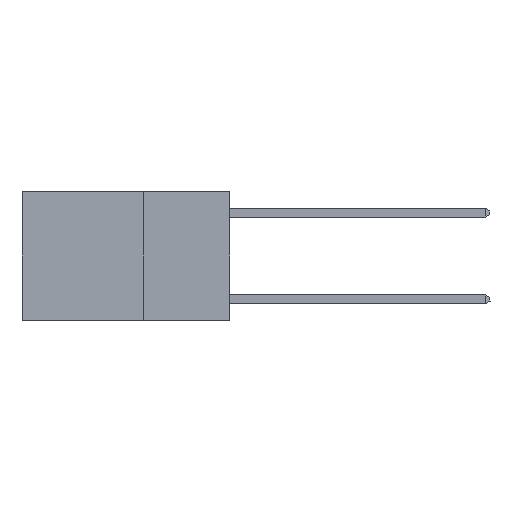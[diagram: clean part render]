
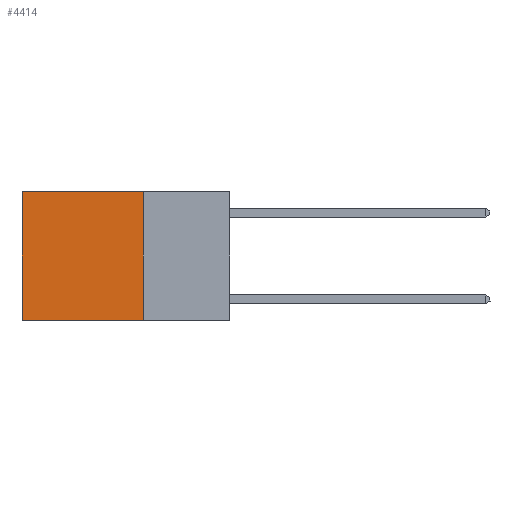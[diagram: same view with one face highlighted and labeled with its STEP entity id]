
A CAD part, left-side view. The second image highlights one B-rep face of the part: STEP entity #4414.
In plain terms, the highlighted planar face has unit normal (-1, 0, 0).
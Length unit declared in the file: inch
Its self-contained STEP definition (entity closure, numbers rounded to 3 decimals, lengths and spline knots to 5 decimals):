
#2287 = EDGE_CURVE ( 'NONE', #24122, #11270, #14135, .T. ) ;
#2678 = EDGE_CURVE ( 'NONE', #27403, #24122, #9421, .T. ) ;
#4101 = AXIS2_PLACEMENT_3D ( 'NONE', #6440, #26783, #15635 ) ;
#4414 = ADVANCED_FACE ( 'NONE', ( #10838 ), #17361, .F. ) ;
#4467 = VECTOR ( 'NONE', #24003, 39.37008 ) ;
#6440 = CARTESIAN_POINT ( 'NONE',  ( 0.2625, 0.25, 0. ) ) ;
#7642 = CARTESIAN_POINT ( 'NONE',  ( 0.2625, 0.25, 0. ) ) ;
#7961 = CARTESIAN_POINT ( 'NONE',  ( 0.2625, 0.6, 0. ) ) ;
#8773 = CARTESIAN_POINT ( 'NONE',  ( 0.2625, 0.25, -0.37 ) ) ;
#9421 = LINE ( 'NONE', #28449, #4467 ) ;
#10534 = EDGE_CURVE ( 'NONE', #18274, #11270, #14956, .T. ) ;
#10838 = FACE_OUTER_BOUND ( 'NONE', #27729, .T. ) ;
#11270 = VERTEX_POINT ( 'NONE', #27602 ) ;
#12934 = LINE ( 'NONE', #20605, #22200 ) ;
#14135 = LINE ( 'NONE', #8773, #26970 ) ;
#14956 = LINE ( 'NONE', #7961, #27405 ) ;
#15513 = ORIENTED_EDGE ( 'NONE', *, *, #2678, .F. ) ;
#15635 = DIRECTION ( 'NONE',  ( 0., 0., -1. ) ) ;
#16086 = DIRECTION ( 'NONE',  ( 0., 1., 0. ) ) ;
#17361 = PLANE ( 'NONE',  #4101 ) ;
#18274 = VERTEX_POINT ( 'NONE', #22081 ) ;
#20605 = CARTESIAN_POINT ( 'NONE',  ( 0.2625, 0.25, 0. ) ) ;
#20937 = ORIENTED_EDGE ( 'NONE', *, *, #10534, .T. ) ;
#22081 = CARTESIAN_POINT ( 'NONE',  ( 0.2625, 0.6, 0. ) ) ;
#22200 = VECTOR ( 'NONE', #16086, 39.37008 ) ;
#23156 = EDGE_CURVE ( 'NONE', #27403, #18274, #12934, .T. ) ;
#24003 = DIRECTION ( 'NONE',  ( 0., 0., -1. ) ) ;
#24122 = VERTEX_POINT ( 'NONE', #26288 ) ;
#24242 = DIRECTION ( 'NONE',  ( 0., 0., -1. ) ) ;
#26138 = ORIENTED_EDGE ( 'NONE', *, *, #2287, .F. ) ;
#26288 = CARTESIAN_POINT ( 'NONE',  ( 0.2625, 0.25, -0.37 ) ) ;
#26783 = DIRECTION ( 'NONE',  ( 1., 0., 0. ) ) ;
#26970 = VECTOR ( 'NONE', #29508, 39.37008 ) ;
#27403 = VERTEX_POINT ( 'NONE', #7642 ) ;
#27405 = VECTOR ( 'NONE', #24242, 39.37008 ) ;
#27602 = CARTESIAN_POINT ( 'NONE',  ( 0.2625, 0.6, -0.37 ) ) ;
#27729 = EDGE_LOOP ( 'NONE', ( #20937, #26138, #15513, #29144 ) ) ;
#28449 = CARTESIAN_POINT ( 'NONE',  ( 0.2625, 0.25, 0. ) ) ;
#29144 = ORIENTED_EDGE ( 'NONE', *, *, #23156, .T. ) ;
#29508 = DIRECTION ( 'NONE',  ( 0., 1., 0. ) ) ;
